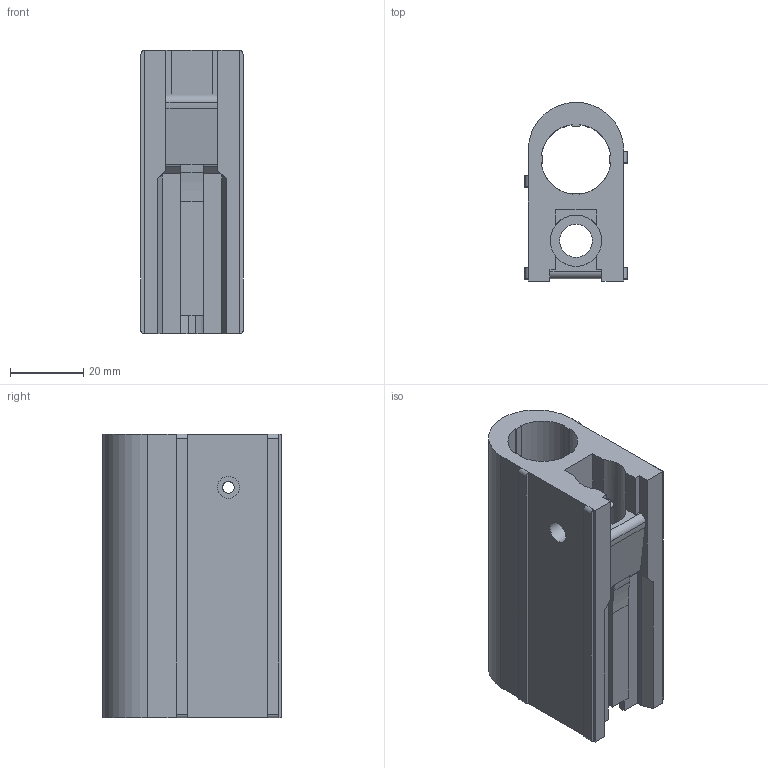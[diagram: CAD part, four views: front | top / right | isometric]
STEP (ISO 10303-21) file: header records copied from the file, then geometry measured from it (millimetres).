
FILE_DESCRIPTION(/* description */ (''),/* implementation_level */ '2;1');
FILE_NAME(/* name */ 'Bolt Housing.step',/* time_stamp */ '2022-05-11T21:16:35-06:00',/* author */ (''),/* organization */ (''),/* preprocessor_version */ 'ST-DEVELOPER v18.1',/* originating_system */ 'Autodesk Translation Framework v10.10.0.1391',/* authorisation */ '');
FILE_SCHEMA (('AUTOMOTIVE_DESIGN { 1 0 10303 214 3 1 1 }'));
Length unit declared in the file: millimetre
Products named in the file (1): Bolt Housing
Bounding box: 27.82 x 48.67 x 77.19 mm (x, y, z)
Volume: 45816 mm3; surface area: 21201.5 mm2
Topology: 1 solids, 1 shells, 98 faces, 269 edges, 174 vertices
Faces by surface type: plane 70, cylinder 28
Full cylindrical faces by diameter (mm): 3.2 x2, 6 x1, 9 x1, 9.5 x1, 14 x1
Entity records: 3207 total; most frequent: CARTESIAN_POINT 614, ORIENTED_EDGE 538, DIRECTION 525, EDGE_CURVE 269, LINE 203, VECTOR 203, VERTEX_POINT 174, AXIS2_PLACEMENT_3D 161
